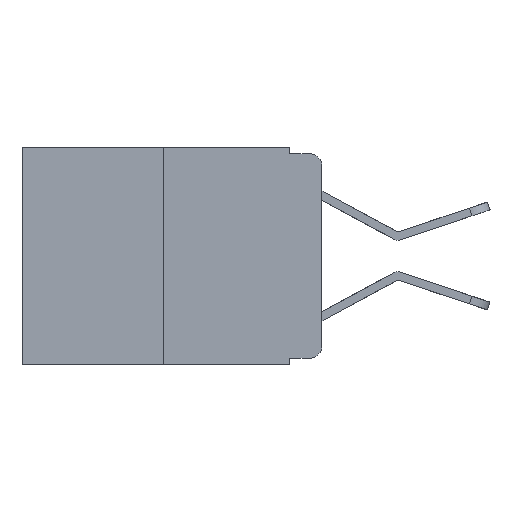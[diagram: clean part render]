
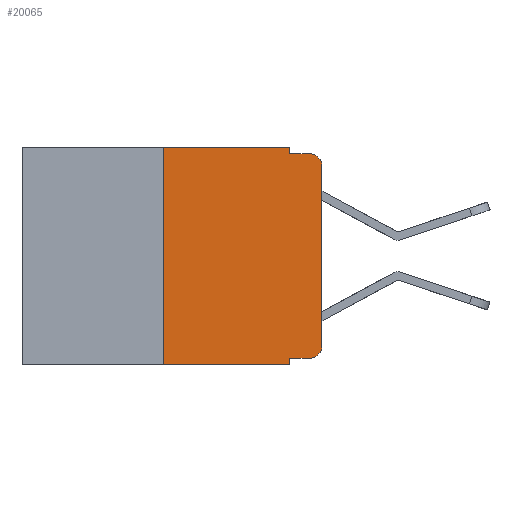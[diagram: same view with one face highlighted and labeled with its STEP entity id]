
A CAD part, left-side view. The second image highlights one B-rep face of the part: STEP entity #20065.
In plain terms, the highlighted planar face has unit normal (-1, 0, 0).
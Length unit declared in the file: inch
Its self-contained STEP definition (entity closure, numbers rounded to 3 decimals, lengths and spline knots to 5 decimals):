
#52 = VERTEX_POINT ( 'NONE', #6103 ) ;
#341 = FACE_OUTER_BOUND ( 'NONE', #19642, .T. ) ;
#420 = CIRCLE ( 'NONE', #5301, 0.02 ) ;
#437 = CARTESIAN_POINT ( 'NONE',  ( 0., 0.051, -0.333 ) ) ;
#656 = LINE ( 'NONE', #19059, #14103 ) ;
#821 = DIRECTION ( 'NONE',  ( 0., -1., 0. ) ) ;
#1646 = DIRECTION ( 'NONE',  ( 0., 0., -1. ) ) ;
#1732 = CARTESIAN_POINT ( 'NONE',  ( 0., 0.473, 0. ) ) ;
#1768 = EDGE_CURVE ( 'NONE', #24228, #4938, #16194, .T. ) ;
#2129 = DIRECTION ( 'NONE',  ( 0., 0., -1. ) ) ;
#2343 = CARTESIAN_POINT ( 'NONE',  ( 0., 0.473, 0. ) ) ;
#2433 = CARTESIAN_POINT ( 'NONE',  ( 0., 0.25, 0. ) ) ;
#2548 = DIRECTION ( 'NONE',  ( 0., 0., 1. ) ) ;
#2595 = LINE ( 'NONE', #437, #23187 ) ;
#2666 = VERTEX_POINT ( 'NONE', #2686 ) ;
#2686 = CARTESIAN_POINT ( 'NONE',  ( 0., 0., -0.03 ) ) ;
#3011 = ORIENTED_EDGE ( 'NONE', *, *, #15857, .F. ) ;
#3594 = DIRECTION ( 'NONE',  ( 0., -1., 0. ) ) ;
#3707 = DIRECTION ( 'NONE',  ( 0., -1., 0. ) ) ;
#3800 = CARTESIAN_POINT ( 'NONE',  ( 0., 0.051, -0.333 ) ) ;
#4803 = VECTOR ( 'NONE', #3594, 39.37008 ) ;
#4804 = VECTOR ( 'NONE', #23461, 39.37008 ) ;
#4938 = VERTEX_POINT ( 'NONE', #11570 ) ;
#5301 = AXIS2_PLACEMENT_3D ( 'NONE', #25211, #5339, #1646 ) ;
#5339 = DIRECTION ( 'NONE',  ( -1., 0., 0. ) ) ;
#6103 = CARTESIAN_POINT ( 'NONE',  ( 0., 0.02, -0.333 ) ) ;
#6147 = DIRECTION ( 'NONE',  ( 0., 0., -1. ) ) ;
#7107 = ORIENTED_EDGE ( 'NONE', *, *, #14077, .T. ) ;
#7180 = VERTEX_POINT ( 'NONE', #10142 ) ;
#7896 = CARTESIAN_POINT ( 'NONE',  ( 0., 0.25, -0.343 ) ) ;
#7914 = ORIENTED_EDGE ( 'NONE', *, *, #17633, .F. ) ;
#7970 = DIRECTION ( 'NONE',  ( 0., 0., -1. ) ) ;
#7971 = ORIENTED_EDGE ( 'NONE', *, *, #20786, .T. ) ;
#8927 = CARTESIAN_POINT ( 'NONE',  ( 0., 0.051, -0.01 ) ) ;
#10014 = PLANE ( 'NONE',  #15919 ) ;
#10142 = CARTESIAN_POINT ( 'NONE',  ( 0., 0., -0.313 ) ) ;
#10152 = CARTESIAN_POINT ( 'NONE',  ( 0., 0.051, 0. ) ) ;
#10188 = AXIS2_PLACEMENT_3D ( 'NONE', #19474, #17933, #6147 ) ;
#10785 = ORIENTED_EDGE ( 'NONE', *, *, #1768, .F. ) ;
#10942 = VERTEX_POINT ( 'NONE', #21907 ) ;
#11537 = DIRECTION ( 'NONE',  ( 0., 0., -1. ) ) ;
#11570 = CARTESIAN_POINT ( 'NONE',  ( 0., 0.051, -0.343 ) ) ;
#11688 = ORIENTED_EDGE ( 'NONE', *, *, #16055, .T. ) ;
#12250 = CIRCLE ( 'NONE', #10188, 0.02 ) ;
#12909 = LINE ( 'NONE', #20864, #4803 ) ;
#13218 = LINE ( 'NONE', #21038, #19040 ) ;
#13417 = VERTEX_POINT ( 'NONE', #7896 ) ;
#13476 = CARTESIAN_POINT ( 'NONE',  ( 0., 0.051, 0. ) ) ;
#13585 = LINE ( 'NONE', #2343, #4804 ) ;
#13833 = VERTEX_POINT ( 'NONE', #14953 ) ;
#14022 = VERTEX_POINT ( 'NONE', #21232 ) ;
#14077 = EDGE_CURVE ( 'NONE', #13417, #4938, #656, .T. ) ;
#14103 = VECTOR ( 'NONE', #3707, 39.37008 ) ;
#14953 = CARTESIAN_POINT ( 'NONE',  ( 0., 0.25, 0. ) ) ;
#15727 = ORIENTED_EDGE ( 'NONE', *, *, #19022, .F. ) ;
#15857 = EDGE_CURVE ( 'NONE', #10942, #23669, #17572, .T. ) ;
#15919 = AXIS2_PLACEMENT_3D ( 'NONE', #1732, #23260, #7970 ) ;
#16055 = EDGE_CURVE ( 'NONE', #24228, #52, #2595, .T. ) ;
#16194 = LINE ( 'NONE', #10152, #21965 ) ;
#17572 = LINE ( 'NONE', #13476, #18683 ) ;
#17633 = EDGE_CURVE ( 'NONE', #13833, #10942, #13585, .T. ) ;
#17719 = ORIENTED_EDGE ( 'NONE', *, *, #22129, .T. ) ;
#17933 = DIRECTION ( 'NONE',  ( -1., 0., 0. ) ) ;
#18293 = LINE ( 'NONE', #2433, #19147 ) ;
#18683 = VECTOR ( 'NONE', #11537, 39.37008 ) ;
#19022 = EDGE_CURVE ( 'NONE', #23669, #14022, #12909, .T. ) ;
#19040 = VECTOR ( 'NONE', #20791, 39.37008 ) ;
#19059 = CARTESIAN_POINT ( 'NONE',  ( 0., 0.473, -0.343 ) ) ;
#19147 = VECTOR ( 'NONE', #2548, 39.37008 ) ;
#19474 = CARTESIAN_POINT ( 'NONE',  ( 0., 0.02, -0.03 ) ) ;
#19642 = EDGE_LOOP ( 'NONE', ( #21874, #17719, #15727, #3011, #7914, #20763, #7107, #10785, #11688, #7971 ) ) ;
#20065 = ADVANCED_FACE ( 'NONE', ( #341 ), #10014, .F. ) ;
#20763 = ORIENTED_EDGE ( 'NONE', *, *, #23927, .F. ) ;
#20786 = EDGE_CURVE ( 'NONE', #52, #7180, #420, .T. ) ;
#20791 = DIRECTION ( 'NONE',  ( 0., 0., 1. ) ) ;
#20864 = CARTESIAN_POINT ( 'NONE',  ( 0., 0.051, -0.01 ) ) ;
#21038 = CARTESIAN_POINT ( 'NONE',  ( 0., 0., 0. ) ) ;
#21232 = CARTESIAN_POINT ( 'NONE',  ( 0., 0.02, -0.01 ) ) ;
#21874 = ORIENTED_EDGE ( 'NONE', *, *, #24642, .T. ) ;
#21907 = CARTESIAN_POINT ( 'NONE',  ( 0., 0.051, 0. ) ) ;
#21965 = VECTOR ( 'NONE', #2129, 39.37008 ) ;
#22129 = EDGE_CURVE ( 'NONE', #2666, #14022, #12250, .T. ) ;
#23187 = VECTOR ( 'NONE', #821, 39.37008 ) ;
#23260 = DIRECTION ( 'NONE',  ( 1., 0., 0. ) ) ;
#23461 = DIRECTION ( 'NONE',  ( 0., -1., 0. ) ) ;
#23669 = VERTEX_POINT ( 'NONE', #8927 ) ;
#23927 = EDGE_CURVE ( 'NONE', #13417, #13833, #18293, .T. ) ;
#24228 = VERTEX_POINT ( 'NONE', #3800 ) ;
#24642 = EDGE_CURVE ( 'NONE', #7180, #2666, #13218, .T. ) ;
#25211 = CARTESIAN_POINT ( 'NONE',  ( 0., 0.02, -0.313 ) ) ;
